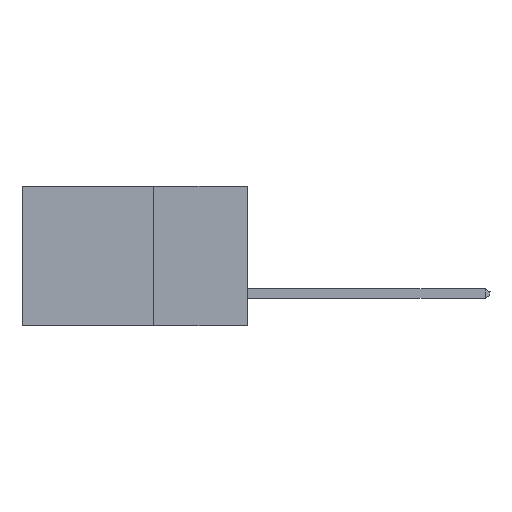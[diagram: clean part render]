
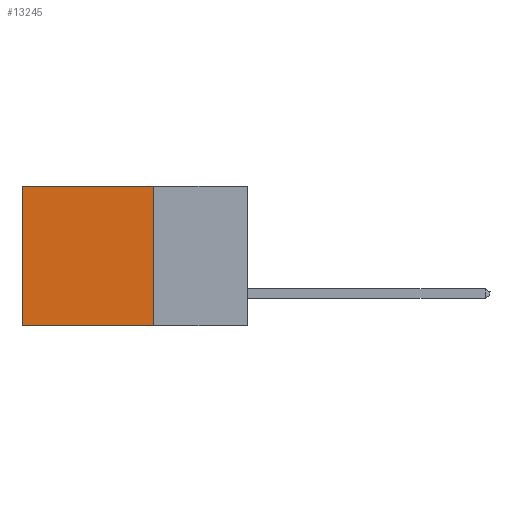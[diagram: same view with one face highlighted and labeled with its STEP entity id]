
A CAD part, left-side view. The second image highlights one B-rep face of the part: STEP entity #13245.
In plain terms, the highlighted planar face has unit normal (-1, 0, 0).
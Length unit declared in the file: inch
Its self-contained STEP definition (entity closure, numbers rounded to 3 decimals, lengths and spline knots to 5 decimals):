
#1287 = ORIENTED_EDGE ( 'NONE', *, *, #4923, .T. ) ;
#1546 = CARTESIAN_POINT ( 'NONE',  ( 0.2615, 0.25, -0.37 ) ) ;
#1652 = DIRECTION ( 'NONE',  ( 1., 0., 0. ) ) ;
#2801 = CARTESIAN_POINT ( 'NONE',  ( 0.2615, 0.25, -0.37 ) ) ;
#2870 = EDGE_CURVE ( 'NONE', #3326, #12284, #12981, .T. ) ;
#3051 = VECTOR ( 'NONE', #7784, 39.37008 ) ;
#3131 = EDGE_LOOP ( 'NONE', ( #4352, #12895, #12857, #1287 ) ) ;
#3326 = VERTEX_POINT ( 'NONE', #4789 ) ;
#3390 = AXIS2_PLACEMENT_3D ( 'NONE', #3947, #1652, #10349 ) ;
#3447 = CARTESIAN_POINT ( 'NONE',  ( 0.2615, 0.6, -0.37 ) ) ;
#3947 = CARTESIAN_POINT ( 'NONE',  ( 0.2615, 0.25, -0.37 ) ) ;
#4352 = ORIENTED_EDGE ( 'NONE', *, *, #8165, .T. ) ;
#4384 = EDGE_CURVE ( 'NONE', #12284, #5292, #9856, .T. ) ;
#4775 = VERTEX_POINT ( 'NONE', #10100 ) ;
#4789 = CARTESIAN_POINT ( 'NONE',  ( 0.2615, 0.25, 0. ) ) ;
#4923 = EDGE_CURVE ( 'NONE', #3326, #4775, #6151, .T. ) ;
#5292 = VERTEX_POINT ( 'NONE', #3447 ) ;
#5811 = DIRECTION ( 'NONE',  ( 0., 0., -1. ) ) ;
#6147 = FACE_OUTER_BOUND ( 'NONE', #3131, .T. ) ;
#6151 = LINE ( 'NONE', #12239, #9463 ) ;
#7242 = LINE ( 'NONE', #8289, #13485 ) ;
#7784 = DIRECTION ( 'NONE',  ( 0., 1., 0. ) ) ;
#8124 = DIRECTION ( 'NONE',  ( 0., 1., 0. ) ) ;
#8165 = EDGE_CURVE ( 'NONE', #4775, #5292, #7242, .T. ) ;
#8289 = CARTESIAN_POINT ( 'NONE',  ( 0.2615, 0.6, -0.37 ) ) ;
#8855 = CARTESIAN_POINT ( 'NONE',  ( 0.2615, 0.25, -0.37 ) ) ;
#9463 = VECTOR ( 'NONE', #8124, 39.37008 ) ;
#9856 = LINE ( 'NONE', #2801, #3051 ) ;
#10100 = CARTESIAN_POINT ( 'NONE',  ( 0.2615, 0.6, 0. ) ) ;
#10188 = VECTOR ( 'NONE', #5811, 39.37008 ) ;
#10349 = DIRECTION ( 'NONE',  ( 0., 0., -1. ) ) ;
#12239 = CARTESIAN_POINT ( 'NONE',  ( 0.2615, 0.25, 0. ) ) ;
#12284 = VERTEX_POINT ( 'NONE', #1546 ) ;
#12414 = DIRECTION ( 'NONE',  ( 0., 0., -1. ) ) ;
#12857 = ORIENTED_EDGE ( 'NONE', *, *, #2870, .F. ) ;
#12895 = ORIENTED_EDGE ( 'NONE', *, *, #4384, .F. ) ;
#12981 = LINE ( 'NONE', #8855, #10188 ) ;
#13245 = ADVANCED_FACE ( 'NONE', ( #6147 ), #13409, .F. ) ;
#13409 = PLANE ( 'NONE',  #3390 ) ;
#13485 = VECTOR ( 'NONE', #12414, 39.37008 ) ;
